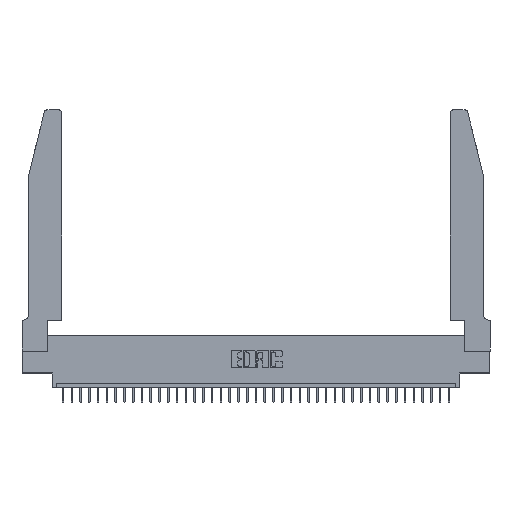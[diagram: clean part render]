
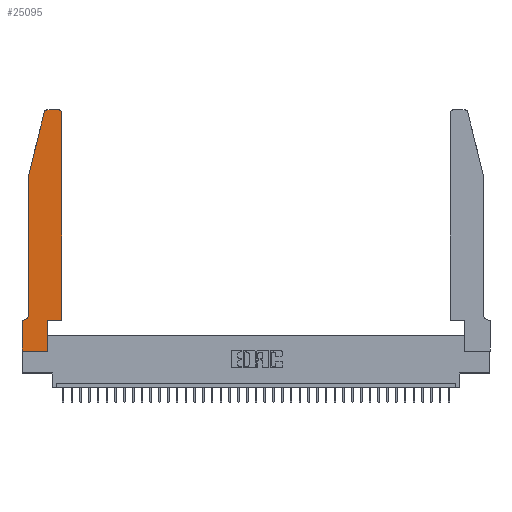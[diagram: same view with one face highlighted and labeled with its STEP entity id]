
A CAD part, top view. The second image highlights one B-rep face of the part: STEP entity #25095.
In plain terms, the highlighted planar face has unit normal (0, 0, 1).
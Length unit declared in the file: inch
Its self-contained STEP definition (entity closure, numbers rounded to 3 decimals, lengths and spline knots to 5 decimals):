
#48 = ORIENTED_EDGE ( 'NONE', *, *, #32748, .T. ) ;
#80 = DIRECTION ( 'NONE',  ( 0., -1., 0. ) ) ;
#600 = EDGE_CURVE ( 'NONE', #27997, #666, #3155, .T. ) ;
#666 = VERTEX_POINT ( 'NONE', #15335 ) ;
#814 = VECTOR ( 'NONE', #14870, 39.37008 ) ;
#1301 = DIRECTION ( 'NONE',  ( 0., 1., 0. ) ) ;
#1818 = DIRECTION ( 'NONE',  ( 0., 1., 0. ) ) ;
#2390 = VERTEX_POINT ( 'NONE', #29799 ) ;
#2462 = VECTOR ( 'NONE', #30123, 39.37008 ) ;
#2808 = CARTESIAN_POINT ( 'NONE',  ( 0.0755, 2., 0.37 ) ) ;
#3155 = LINE ( 'NONE', #9229, #15663 ) ;
#3793 = CARTESIAN_POINT ( 'NONE',  ( 0., 0.35, 0.37 ) ) ;
#4008 = VERTEX_POINT ( 'NONE', #29075 ) ;
#4450 = CARTESIAN_POINT ( 'NONE',  ( 0.4505, 2.72, 0.37 ) ) ;
#4684 = CARTESIAN_POINT ( 'NONE',  ( 0.4205, 2.75, 0.37 ) ) ;
#5139 = ORIENTED_EDGE ( 'NONE', *, *, #20193, .T. ) ;
#5384 = CARTESIAN_POINT ( 'NONE',  ( 0.0755, 0.35, 0.37 ) ) ;
#5626 = DIRECTION ( 'NONE',  ( -0.239, -0.971, 0. ) ) ;
#6068 = CARTESIAN_POINT ( 'NONE',  ( 0., 0., 0.37 ) ) ;
#6206 = EDGE_CURVE ( 'NONE', #29308, #15925, #35044, .T. ) ;
#6705 = CARTESIAN_POINT ( 'NONE',  ( 0.2865, 0.35, 0.37 ) ) ;
#8211 = FACE_OUTER_BOUND ( 'NONE', #20275, .T. ) ;
#8838 = LINE ( 'NONE', #2808, #32548 ) ;
#9212 = EDGE_CURVE ( 'NONE', #666, #18095, #8838, .T. ) ;
#9229 = CARTESIAN_POINT ( 'NONE',  ( 0.0755, 2., 0.37 ) ) ;
#9296 = AXIS2_PLACEMENT_3D ( 'NONE', #10574, #29128, #24523 ) ;
#9346 = VECTOR ( 'NONE', #11327, 39.37008 ) ;
#9488 = VERTEX_POINT ( 'NONE', #13207 ) ;
#9599 = CARTESIAN_POINT ( 'NONE',  ( 0.2865, 0., 0.37 ) ) ;
#9839 = DIRECTION ( 'NONE',  ( -1., 0., 0. ) ) ;
#10021 = ORIENTED_EDGE ( 'NONE', *, *, #10885, .T. ) ;
#10574 = CARTESIAN_POINT ( 'NONE',  ( 0.4205, 2.72, 0.37 ) ) ;
#10885 = EDGE_CURVE ( 'NONE', #18095, #4008, #24858, .T. ) ;
#11327 = DIRECTION ( 'NONE',  ( -1., 0., 0. ) ) ;
#11522 = CARTESIAN_POINT ( 'NONE',  ( 0., 0., 0.37 ) ) ;
#12040 = LINE ( 'NONE', #6068, #34802 ) ;
#12117 = CARTESIAN_POINT ( 'NONE',  ( 0.0755, 0.42, 0.37 ) ) ;
#12366 = CIRCLE ( 'NONE', #20394, 0.03 ) ;
#12485 = VERTEX_POINT ( 'NONE', #4450 ) ;
#13207 = CARTESIAN_POINT ( 'NONE',  ( 0., 0.35, 0.37 ) ) ;
#14870 = DIRECTION ( 'NONE',  ( 0., -1., 0. ) ) ;
#15148 = CIRCLE ( 'NONE', #9296, 0.03 ) ;
#15262 = DIRECTION ( 'NONE',  ( 1., 0., 0. ) ) ;
#15327 = LINE ( 'NONE', #37285, #32077 ) ;
#15335 = CARTESIAN_POINT ( 'NONE',  ( 0.0755, 2., 0.37 ) ) ;
#15528 = VERTEX_POINT ( 'NONE', #21777 ) ;
#15564 = PLANE ( 'NONE',  #29937 ) ;
#15663 = VECTOR ( 'NONE', #5626, 39.37008 ) ;
#15925 = VERTEX_POINT ( 'NONE', #6705 ) ;
#16041 = ORIENTED_EDGE ( 'NONE', *, *, #17510, .T. ) ;
#16532 = CARTESIAN_POINT ( 'NONE',  ( 0.284, 2.75, 0.37 ) ) ;
#16891 = EDGE_CURVE ( 'NONE', #15925, #2390, #24695, .T. ) ;
#17510 = EDGE_CURVE ( 'NONE', #33124, #17556, #15327, .T. ) ;
#17556 = VERTEX_POINT ( 'NONE', #16532 ) ;
#18095 = VERTEX_POINT ( 'NONE', #12117 ) ;
#18186 = CARTESIAN_POINT ( 'NONE',  ( 0.4505, 0.35, 0.37 ) ) ;
#19996 = ORIENTED_EDGE ( 'NONE', *, *, #6206, .T. ) ;
#20193 = EDGE_CURVE ( 'NONE', #9488, #15528, #35617, .T. ) ;
#20275 = EDGE_LOOP ( 'NONE', ( #16041, #48, #20481, #36965, #10021, #32367, #5139, #22831, #19996, #28044, #34010, #24835 ) ) ;
#20394 = AXIS2_PLACEMENT_3D ( 'NONE', #24032, #21138, #36344 ) ;
#20481 = ORIENTED_EDGE ( 'NONE', *, *, #600, .T. ) ;
#20922 = CARTESIAN_POINT ( 'NONE',  ( 0.25487, 2.72718, 0.37 ) ) ;
#21138 = DIRECTION ( 'NONE',  ( 0., 0., 1. ) ) ;
#21640 = CARTESIAN_POINT ( 'NONE',  ( 0.0055, 0.42, 0.37 ) ) ;
#21777 = CARTESIAN_POINT ( 'NONE',  ( 0., 0., 0.37 ) ) ;
#21815 = AXIS2_PLACEMENT_3D ( 'NONE', #21640, #24666, #9839 ) ;
#22747 = VECTOR ( 'NONE', #1818, 39.37008 ) ;
#22768 = DIRECTION ( 'NONE',  ( -1., 0., 0. ) ) ;
#22831 = ORIENTED_EDGE ( 'NONE', *, *, #31632, .T. ) ;
#24032 = CARTESIAN_POINT ( 'NONE',  ( 0.284, 2.72, 0.37 ) ) ;
#24523 = DIRECTION ( 'NONE',  ( 1., 0., 0. ) ) ;
#24666 = DIRECTION ( 'NONE',  ( 0., 0., -1. ) ) ;
#24695 = LINE ( 'NONE', #18186, #2462 ) ;
#24835 = ORIENTED_EDGE ( 'NONE', *, *, #25131, .T. ) ;
#24858 = CIRCLE ( 'NONE', #21815, 0.07 ) ;
#25031 = CARTESIAN_POINT ( 'NONE',  ( 0.2865, 0.35, 0.37 ) ) ;
#25095 = ADVANCED_FACE ( 'NONE', ( #8211 ), #15564, .T. ) ;
#25131 = EDGE_CURVE ( 'NONE', #12485, #33124, #15148, .T. ) ;
#27466 = DIRECTION ( 'NONE',  ( 0., 0., 1. ) ) ;
#27725 = DIRECTION ( 'NONE',  ( 1., 0., 0. ) ) ;
#27997 = VERTEX_POINT ( 'NONE', #20922 ) ;
#28044 = ORIENTED_EDGE ( 'NONE', *, *, #16891, .T. ) ;
#29075 = CARTESIAN_POINT ( 'NONE',  ( 0.0055, 0.35, 0.37 ) ) ;
#29128 = DIRECTION ( 'NONE',  ( 0., 0., 1. ) ) ;
#29308 = VERTEX_POINT ( 'NONE', #9599 ) ;
#29615 = EDGE_CURVE ( 'NONE', #4008, #9488, #34918, .T. ) ;
#29799 = CARTESIAN_POINT ( 'NONE',  ( 0.4505, 0.35, 0.37 ) ) ;
#29937 = AXIS2_PLACEMENT_3D ( 'NONE', #3793, #27466, #27725 ) ;
#30123 = DIRECTION ( 'NONE',  ( 1., 0., 0. ) ) ;
#31328 = EDGE_CURVE ( 'NONE', #2390, #12485, #31570, .T. ) ;
#31570 = LINE ( 'NONE', #31920, #22747 ) ;
#31632 = EDGE_CURVE ( 'NONE', #15528, #29308, #12040, .T. ) ;
#31920 = CARTESIAN_POINT ( 'NONE',  ( 0.4505, 0.35, 0.37 ) ) ;
#32077 = VECTOR ( 'NONE', #22768, 39.37008 ) ;
#32367 = ORIENTED_EDGE ( 'NONE', *, *, #29615, .T. ) ;
#32548 = VECTOR ( 'NONE', #80, 39.37008 ) ;
#32748 = EDGE_CURVE ( 'NONE', #17556, #27997, #12366, .T. ) ;
#33124 = VERTEX_POINT ( 'NONE', #4684 ) ;
#34010 = ORIENTED_EDGE ( 'NONE', *, *, #31328, .T. ) ;
#34802 = VECTOR ( 'NONE', #15262, 39.37008 ) ;
#34918 = LINE ( 'NONE', #5384, #9346 ) ;
#35044 = LINE ( 'NONE', #25031, #36399 ) ;
#35617 = LINE ( 'NONE', #11522, #814 ) ;
#36344 = DIRECTION ( 'NONE',  ( 1., 0., 0. ) ) ;
#36399 = VECTOR ( 'NONE', #1301, 39.37008 ) ;
#36965 = ORIENTED_EDGE ( 'NONE', *, *, #9212, .T. ) ;
#37285 = CARTESIAN_POINT ( 'NONE',  ( 0.2605, 2.75, 0.37 ) ) ;
